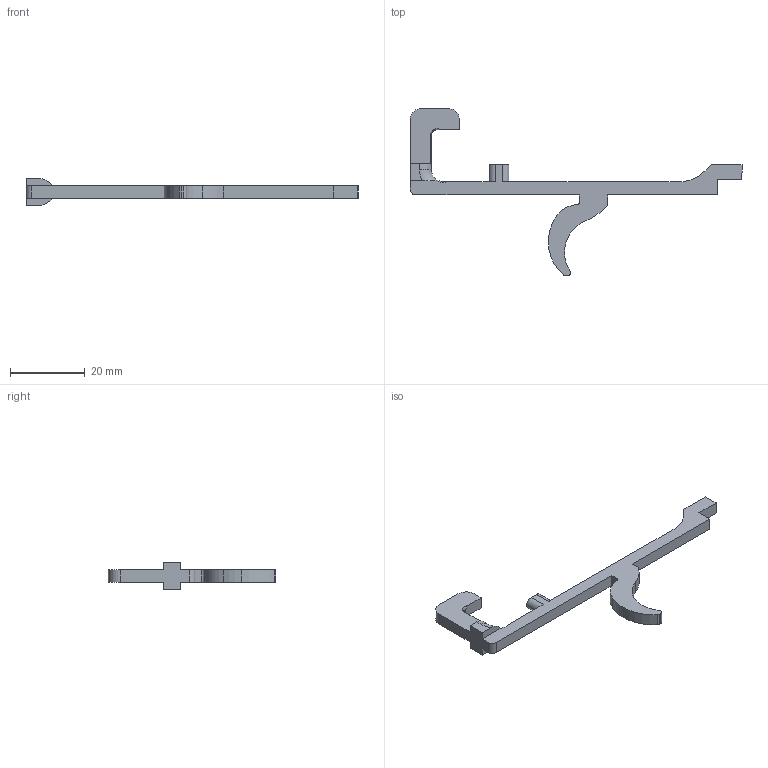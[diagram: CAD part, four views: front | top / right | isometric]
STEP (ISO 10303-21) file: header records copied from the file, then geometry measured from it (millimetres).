
FILE_DESCRIPTION (( 'STEP AP214' ), '1' );
FILE_NAME ('trigger.STEP', '2013-06-07T17:14:51', ( 'Asher' ), ( '' ), 'SwSTEP 2.0', 'SolidWorks 2013', '' );
FILE_SCHEMA (( 'AUTOMOTIVE_DESIGN' ));
Length unit declared in the file: millimetre
Products named in the file (1): trigger
Bounding box: 89.12 x 44.91 x 7.37 mm (x, y, z)
Volume: 2223.2 mm3; surface area: 2334.5 mm2
Topology: 1 solids, 1 shells, 54 faces, 152 edges, 100 vertices
Faces by surface type: plane 29, cylinder 21, torus 4
Entity records: 1806 total; most frequent: CARTESIAN_POINT 337, DIRECTION 306, ORIENTED_EDGE 304, EDGE_CURVE 152, AXIS2_PLACEMENT_3D 105, VERTEX_POINT 100, LINE 96, VECTOR 96
